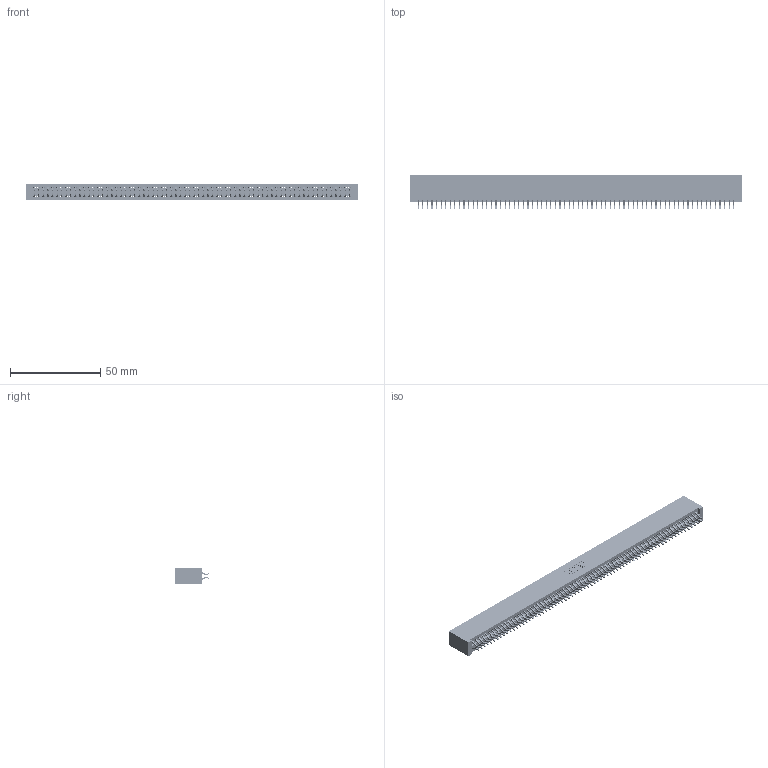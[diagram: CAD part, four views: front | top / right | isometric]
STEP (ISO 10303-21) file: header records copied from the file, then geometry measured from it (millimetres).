
FILE_DESCRIPTION (( 'STEP AP203' ), '1' );
FILE_NAME ('345-140-556-201.STEP', '2019-11-08T22:33:03', ( '' ), ( '' ), 'SwSTEP 2.0', 'SolidWorks 2016', '' );
FILE_SCHEMA (( 'CONFIG_CONTROL_DESIGN' ));
Length unit declared in the file: inch
Products named in the file (3): 345-140-556-201; 345 Part_No Mounting Lugs; 345-292-001_556 Tail
Assembly tree (141 placements, depth 2):
  345-140-556-201
    345 Part_No Mounting Lugs
    345-292-001_556 Tail  x140
Bounding box: 184.4 x 19.24 x 9.4 mm (x, y, z)
Volume: 18783.5 mm3; surface area: 28488.1 mm2
Topology: 141 solids, 141 shells, 7958 faces, 23697 edges, 15610 vertices
Faces by surface type: plane 5256, cylinder 2702
Entity records: 51097 total; most frequent: CARTESIAN_POINT 8552, ORIENTED_EDGE 8474, DIRECTION 7489, EDGE_CURVE 4237, VECTOR 3825, LINE 3825, VERTEX_POINT 2822, AXIS2_PLACEMENT_3D 1832
